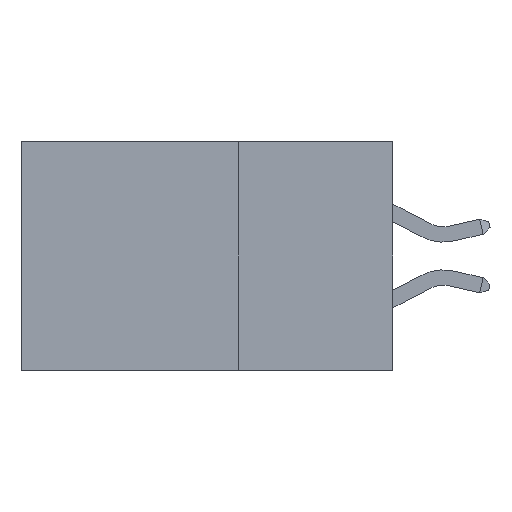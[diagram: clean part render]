
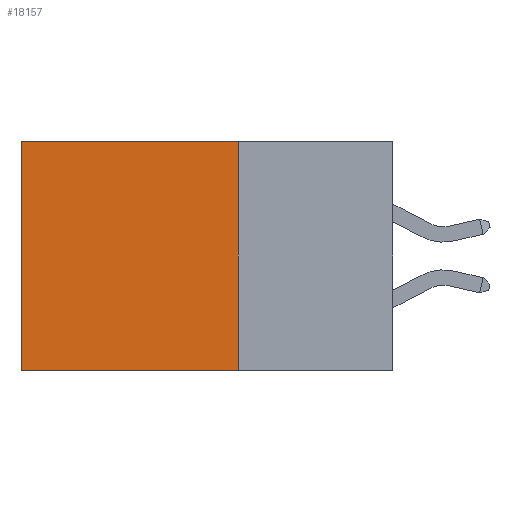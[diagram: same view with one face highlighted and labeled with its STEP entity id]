
A CAD part, left-side view. The second image highlights one B-rep face of the part: STEP entity #18157.
In plain terms, the highlighted planar face has unit normal (-1, 0, 0).
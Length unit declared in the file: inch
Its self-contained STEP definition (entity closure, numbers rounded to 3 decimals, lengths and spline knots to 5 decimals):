
#404 = LINE ( 'NONE', #531, #18001 ) ;
#531 = CARTESIAN_POINT ( 'NONE',  ( 0.2875, 0.25, 0. ) ) ;
#1396 = CARTESIAN_POINT ( 'NONE',  ( 0.2875, 0.25, 0. ) ) ;
#2271 = ORIENTED_EDGE ( 'NONE', *, *, #20431, .F. ) ;
#3221 = PLANE ( 'NONE',  #4028 ) ;
#3227 = EDGE_LOOP ( 'NONE', ( #17612, #11016, #2271, #18120 ) ) ;
#3397 = CARTESIAN_POINT ( 'NONE',  ( 0.2875, 0.6, -0.37 ) ) ;
#3552 = CARTESIAN_POINT ( 'NONE',  ( 0.2875, 0.6, 0. ) ) ;
#3874 = CARTESIAN_POINT ( 'NONE',  ( 0.2875, 0.25, 0. ) ) ;
#4028 = AXIS2_PLACEMENT_3D ( 'NONE', #1396, #7003, #13743 ) ;
#4055 = CARTESIAN_POINT ( 'NONE',  ( 0.2875, 0.25, 0. ) ) ;
#5115 = EDGE_CURVE ( 'NONE', #19637, #16783, #404, .T. ) ;
#5394 = CARTESIAN_POINT ( 'NONE',  ( 0.2875, 0.25, -0.37 ) ) ;
#6262 = VECTOR ( 'NONE', #8415, 39.37008 ) ;
#7003 = DIRECTION ( 'NONE',  ( 1., 0., 0. ) ) ;
#7401 = DIRECTION ( 'NONE',  ( 0., 1., 0. ) ) ;
#8415 = DIRECTION ( 'NONE',  ( 0., 0., -1. ) ) ;
#10812 = VERTEX_POINT ( 'NONE', #3397 ) ;
#11016 = ORIENTED_EDGE ( 'NONE', *, *, #12862, .F. ) ;
#12820 = DIRECTION ( 'NONE',  ( 0., 1., 0. ) ) ;
#12862 = EDGE_CURVE ( 'NONE', #15598, #10812, #16087, .T. ) ;
#12903 = VECTOR ( 'NONE', #16368, 39.37008 ) ;
#12915 = LINE ( 'NONE', #15159, #6262 ) ;
#13501 = EDGE_CURVE ( 'NONE', #16783, #10812, #12915, .T. ) ;
#13743 = DIRECTION ( 'NONE',  ( 0., 0., -1. ) ) ;
#15159 = CARTESIAN_POINT ( 'NONE',  ( 0.2875, 0.6, 0. ) ) ;
#15598 = VERTEX_POINT ( 'NONE', #5394 ) ;
#16087 = LINE ( 'NONE', #19289, #21916 ) ;
#16368 = DIRECTION ( 'NONE',  ( 0., 0., -1. ) ) ;
#16783 = VERTEX_POINT ( 'NONE', #3552 ) ;
#17612 = ORIENTED_EDGE ( 'NONE', *, *, #13501, .T. ) ;
#18001 = VECTOR ( 'NONE', #7401, 39.37008 ) ;
#18120 = ORIENTED_EDGE ( 'NONE', *, *, #5115, .T. ) ;
#18157 = ADVANCED_FACE ( 'NONE', ( #19089 ), #3221, .F. ) ;
#19089 = FACE_OUTER_BOUND ( 'NONE', #3227, .T. ) ;
#19289 = CARTESIAN_POINT ( 'NONE',  ( 0.2875, 0.25, -0.37 ) ) ;
#19637 = VERTEX_POINT ( 'NONE', #3874 ) ;
#19927 = LINE ( 'NONE', #4055, #12903 ) ;
#20431 = EDGE_CURVE ( 'NONE', #19637, #15598, #19927, .T. ) ;
#21916 = VECTOR ( 'NONE', #12820, 39.37008 ) ;
